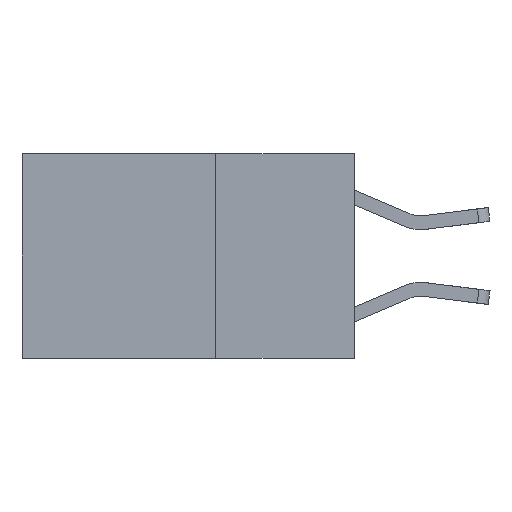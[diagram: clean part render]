
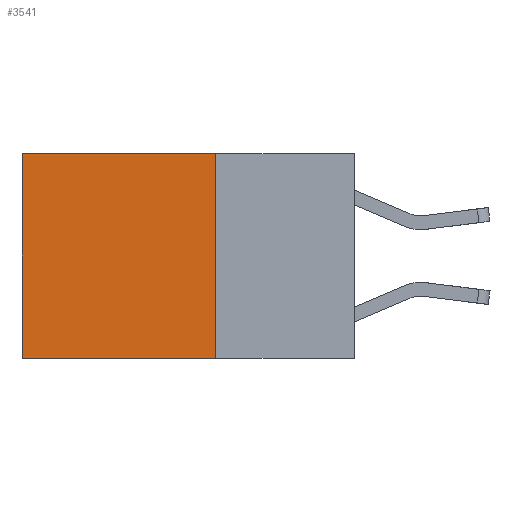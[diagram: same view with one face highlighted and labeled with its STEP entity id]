
A CAD part, left-side view. The second image highlights one B-rep face of the part: STEP entity #3541.
In plain terms, the highlighted planar face has unit normal (-1, 0, 0).
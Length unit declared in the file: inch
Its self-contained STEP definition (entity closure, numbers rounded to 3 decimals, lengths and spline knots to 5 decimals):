
#34 = EDGE_LOOP ( 'NONE', ( #383, #1510, #3872, #958 ) ) ;
#244 = CARTESIAN_POINT ( 'NONE',  ( 0.2625, 0.6, 0. ) ) ;
#383 = ORIENTED_EDGE ( 'NONE', *, *, #2830, .T. ) ;
#560 = VECTOR ( 'NONE', #2294, 39.37008 ) ;
#958 = ORIENTED_EDGE ( 'NONE', *, *, #8510, .T. ) ;
#1054 = AXIS2_PLACEMENT_3D ( 'NONE', #10095, #4896, #10949 ) ;
#1182 = VERTEX_POINT ( 'NONE', #9842 ) ;
#1354 = LINE ( 'NONE', #11296, #2902 ) ;
#1448 = CARTESIAN_POINT ( 'NONE',  ( 0.2625, 0.6, -0.37 ) ) ;
#1510 = ORIENTED_EDGE ( 'NONE', *, *, #6452, .F. ) ;
#2294 = DIRECTION ( 'NONE',  ( 0., 1., 0. ) ) ;
#2332 = FACE_OUTER_BOUND ( 'NONE', #34, .T. ) ;
#2660 = LINE ( 'NONE', #7566, #560 ) ;
#2830 = EDGE_CURVE ( 'NONE', #10224, #5871, #4006, .T. ) ;
#2902 = VECTOR ( 'NONE', #3486, 39.37008 ) ;
#3486 = DIRECTION ( 'NONE',  ( 0., 1., 0. ) ) ;
#3541 = ADVANCED_FACE ( 'NONE', ( #2332 ), #8376, .F. ) ;
#3610 = EDGE_CURVE ( 'NONE', #9237, #1182, #5945, .T. ) ;
#3872 = ORIENTED_EDGE ( 'NONE', *, *, #3610, .F. ) ;
#4006 = LINE ( 'NONE', #244, #6098 ) ;
#4896 = DIRECTION ( 'NONE',  ( 1., 0., 0. ) ) ;
#5777 = CARTESIAN_POINT ( 'NONE',  ( 0.2625, 0.6, 0. ) ) ;
#5871 = VERTEX_POINT ( 'NONE', #1448 ) ;
#5945 = LINE ( 'NONE', #7618, #10241 ) ;
#6098 = VECTOR ( 'NONE', #7333, 39.37008 ) ;
#6452 = EDGE_CURVE ( 'NONE', #1182, #5871, #2660, .T. ) ;
#7055 = CARTESIAN_POINT ( 'NONE',  ( 0.2625, 0.25, 0. ) ) ;
#7333 = DIRECTION ( 'NONE',  ( 0., 0., -1. ) ) ;
#7566 = CARTESIAN_POINT ( 'NONE',  ( 0.2625, 0.25, -0.37 ) ) ;
#7618 = CARTESIAN_POINT ( 'NONE',  ( 0.2625, 0.25, 0. ) ) ;
#8376 = PLANE ( 'NONE',  #1054 ) ;
#8495 = DIRECTION ( 'NONE',  ( 0., 0., -1. ) ) ;
#8510 = EDGE_CURVE ( 'NONE', #9237, #10224, #1354, .T. ) ;
#9237 = VERTEX_POINT ( 'NONE', #7055 ) ;
#9842 = CARTESIAN_POINT ( 'NONE',  ( 0.2625, 0.25, -0.37 ) ) ;
#10095 = CARTESIAN_POINT ( 'NONE',  ( 0.2625, 0.25, 0. ) ) ;
#10224 = VERTEX_POINT ( 'NONE', #5777 ) ;
#10241 = VECTOR ( 'NONE', #8495, 39.37008 ) ;
#10949 = DIRECTION ( 'NONE',  ( 0., 0., -1. ) ) ;
#11296 = CARTESIAN_POINT ( 'NONE',  ( 0.2625, 0.25, 0. ) ) ;
